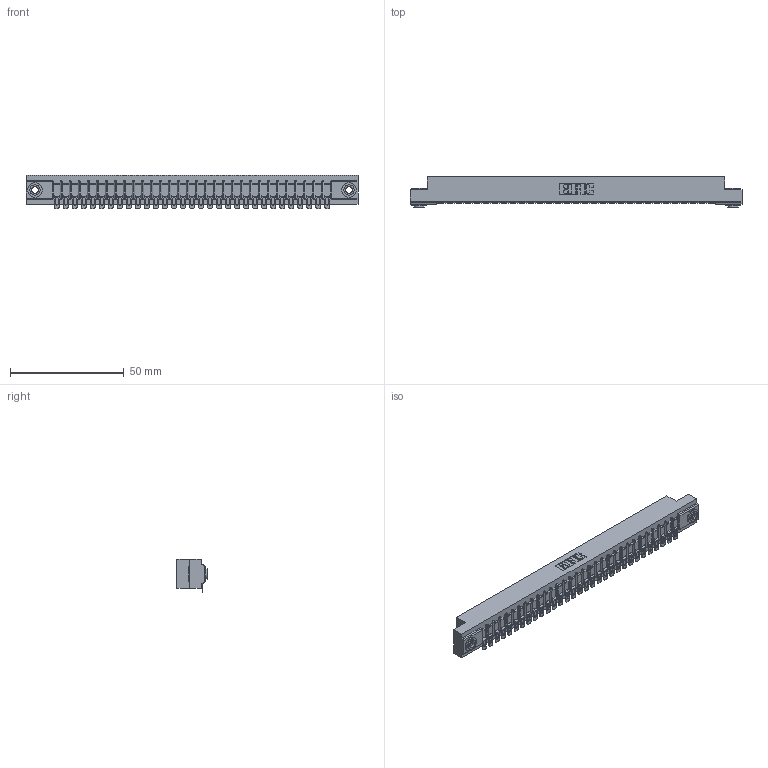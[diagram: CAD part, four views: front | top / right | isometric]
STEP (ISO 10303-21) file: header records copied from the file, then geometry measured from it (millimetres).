
FILE_DESCRIPTION (( 'STEP AP203' ), '1' );
FILE_NAME ('357-031-554-103.STEP', '2019-09-17T03:53:31', ( '' ), ( '' ), 'SwSTEP 2.0', 'SolidWorks 2016', '' );
FILE_SCHEMA (( 'CONFIG_CONTROL_DESIGN' ));
Length unit declared in the file: inch
Products named in the file (4): 307-290-002_554; 307 Part_.156 Dia Mounting Holes; 357-031-554-103; 345-250-002_345-250-002-102
Assembly tree (34 placements, depth 2):
  357-031-554-103
    307 Part_.156 Dia Mounting Holes
    307-290-002_554  x31
    345-250-002_345-250-002-102  x2
Bounding box: 145.85 x 13.36 x 14.52 mm (x, y, z)
Volume: 15537.9 mm3; surface area: 19664.5 mm2
Topology: 34 solids, 34 shells, 2713 faces, 8278 edges, 5428 vertices
Faces by surface type: plane 1520, cylinder 1121, sphere 64, cone 8
Entity records: 29962 total; most frequent: CARTESIAN_POINT 5031, ORIENTED_EDGE 5012, DIRECTION 4914, EDGE_CURVE 2506, LINE 1900, VECTOR 1900, VERTEX_POINT 1624, AXIS2_PLACEMENT_3D 1507
